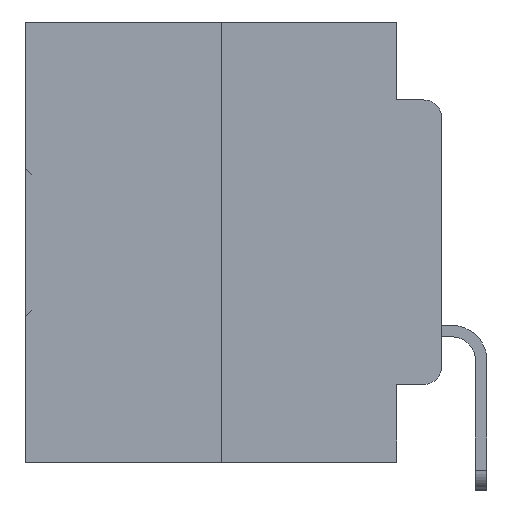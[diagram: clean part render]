
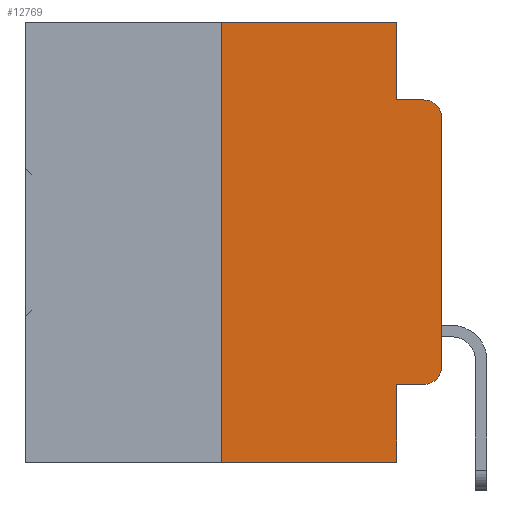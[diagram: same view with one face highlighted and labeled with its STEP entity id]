
A CAD part, left-side view. The second image highlights one B-rep face of the part: STEP entity #12769.
In plain terms, the highlighted planar face has unit normal (-1, 0, 0).
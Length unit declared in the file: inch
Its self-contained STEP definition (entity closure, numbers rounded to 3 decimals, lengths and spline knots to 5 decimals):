
#136 = CARTESIAN_POINT ( 'NONE',  ( 0., 0.02, -0.1085 ) ) ;
#420 = VECTOR ( 'NONE', #32712, 39.37008 ) ;
#559 = LINE ( 'NONE', #23580, #27703 ) ;
#702 = EDGE_CURVE ( 'NONE', #16581, #24952, #32642, .T. ) ;
#1032 = VERTEX_POINT ( 'NONE', #11957 ) ;
#1136 = CARTESIAN_POINT ( 'NONE',  ( 0., 0.02, -0.3915 ) ) ;
#1453 = ORIENTED_EDGE ( 'NONE', *, *, #24334, .T. ) ;
#2883 = DIRECTION ( 'NONE',  ( 0., 0., -1. ) ) ;
#3079 = ORIENTED_EDGE ( 'NONE', *, *, #13351, .F. ) ;
#3846 = DIRECTION ( 'NONE',  ( 0., 0., -1. ) ) ;
#4334 = EDGE_CURVE ( 'NONE', #1032, #16581, #8458, .T. ) ;
#4738 = EDGE_CURVE ( 'NONE', #27510, #22793, #20989, .T. ) ;
#4825 = EDGE_LOOP ( 'NONE', ( #1453, #26632, #18326, #22467, #15702, #8061, #13616, #3079, #13171, #13235 ) ) ;
#5275 = VECTOR ( 'NONE', #8597, 39.37008 ) ;
#6182 = VECTOR ( 'NONE', #15870, 39.37008 ) ;
#6198 = CARTESIAN_POINT ( 'NONE',  ( 0., 0.473, 0. ) ) ;
#6335 = AXIS2_PLACEMENT_3D ( 'NONE', #136, #18748, #2883 ) ;
#6555 = CARTESIAN_POINT ( 'NONE',  ( 0., 0.02, -0.0885 ) ) ;
#7232 = DIRECTION ( 'NONE',  ( 0., -1., 0. ) ) ;
#7271 = LINE ( 'NONE', #9336, #18768 ) ;
#7338 = LINE ( 'NONE', #14507, #20489 ) ;
#7946 = EDGE_CURVE ( 'NONE', #31544, #31928, #7271, .T. ) ;
#8061 = ORIENTED_EDGE ( 'NONE', *, *, #7946, .F. ) ;
#8458 = LINE ( 'NONE', #33052, #420 ) ;
#8597 = DIRECTION ( 'NONE',  ( 0., 0., -1. ) ) ;
#8681 = FACE_OUTER_BOUND ( 'NONE', #4825, .T. ) ;
#8871 = PLANE ( 'NONE',  #21609 ) ;
#9336 = CARTESIAN_POINT ( 'NONE',  ( 0., 0.25, 0. ) ) ;
#11580 = CARTESIAN_POINT ( 'NONE',  ( 0., 0.25, -0.5 ) ) ;
#11719 = CARTESIAN_POINT ( 'NONE',  ( 0., 0.02, -0.4115 ) ) ;
#11918 = AXIS2_PLACEMENT_3D ( 'NONE', #1136, #19691, #3846 ) ;
#11957 = CARTESIAN_POINT ( 'NONE',  ( 0., 0.051, 0. ) ) ;
#12186 = CARTESIAN_POINT ( 'NONE',  ( 0., 0., -0.1085 ) ) ;
#12450 = LINE ( 'NONE', #13882, #5275 ) ;
#12769 = ADVANCED_FACE ( 'NONE', ( #8681 ), #8871, .F. ) ;
#13171 = ORIENTED_EDGE ( 'NONE', *, *, #4738, .T. ) ;
#13235 = ORIENTED_EDGE ( 'NONE', *, *, #17181, .T. ) ;
#13351 = EDGE_CURVE ( 'NONE', #27510, #23651, #12450, .T. ) ;
#13353 = DIRECTION ( 'NONE',  ( 0., -1., 0. ) ) ;
#13616 = ORIENTED_EDGE ( 'NONE', *, *, #30329, .T. ) ;
#13882 = CARTESIAN_POINT ( 'NONE',  ( 0., 0.051, 0. ) ) ;
#14507 = CARTESIAN_POINT ( 'NONE',  ( 0., 0., 0. ) ) ;
#15702 = ORIENTED_EDGE ( 'NONE', *, *, #25125, .F. ) ;
#15870 = DIRECTION ( 'NONE',  ( 0., -1., 0. ) ) ;
#15890 = CARTESIAN_POINT ( 'NONE',  ( 0., 0.051, -0.4115 ) ) ;
#16581 = VERTEX_POINT ( 'NONE', #18728 ) ;
#16833 = DIRECTION ( 'NONE',  ( 0., 0., -1. ) ) ;
#17181 = EDGE_CURVE ( 'NONE', #22793, #25713, #19619, .T. ) ;
#17774 = VERTEX_POINT ( 'NONE', #12186 ) ;
#18326 = ORIENTED_EDGE ( 'NONE', *, *, #702, .F. ) ;
#18613 = CIRCLE ( 'NONE', #6335, 0.02 ) ;
#18728 = CARTESIAN_POINT ( 'NONE',  ( 0., 0.051, -0.0885 ) ) ;
#18748 = DIRECTION ( 'NONE',  ( -1., 0., 0. ) ) ;
#18768 = VECTOR ( 'NONE', #27503, 39.37008 ) ;
#19619 = CIRCLE ( 'NONE', #11918, 0.02 ) ;
#19691 = DIRECTION ( 'NONE',  ( -1., 0., 0. ) ) ;
#19696 = DIRECTION ( 'NONE',  ( 0., 0., 1. ) ) ;
#20489 = VECTOR ( 'NONE', #19696, 39.37008 ) ;
#20989 = LINE ( 'NONE', #15890, #6182 ) ;
#21609 = AXIS2_PLACEMENT_3D ( 'NONE', #6198, #32214, #16833 ) ;
#22467 = ORIENTED_EDGE ( 'NONE', *, *, #4334, .F. ) ;
#22793 = VERTEX_POINT ( 'NONE', #11719 ) ;
#23580 = CARTESIAN_POINT ( 'NONE',  ( 0., 0.473, -0.5 ) ) ;
#23651 = VERTEX_POINT ( 'NONE', #29346 ) ;
#24334 = EDGE_CURVE ( 'NONE', #25713, #17774, #7338, .T. ) ;
#24829 = DIRECTION ( 'NONE',  ( 0., -1., 0. ) ) ;
#24952 = VERTEX_POINT ( 'NONE', #6555 ) ;
#25125 = EDGE_CURVE ( 'NONE', #31928, #1032, #30451, .T. ) ;
#25713 = VERTEX_POINT ( 'NONE', #26547 ) ;
#25841 = VECTOR ( 'NONE', #24829, 39.37008 ) ;
#25899 = CARTESIAN_POINT ( 'NONE',  ( 0., 0.25, 0. ) ) ;
#26359 = CARTESIAN_POINT ( 'NONE',  ( 0., 0.051, -0.0885 ) ) ;
#26547 = CARTESIAN_POINT ( 'NONE',  ( 0., 0., -0.3915 ) ) ;
#26632 = ORIENTED_EDGE ( 'NONE', *, *, #27778, .T. ) ;
#27503 = DIRECTION ( 'NONE',  ( 0., 0., 1. ) ) ;
#27510 = VERTEX_POINT ( 'NONE', #27879 ) ;
#27703 = VECTOR ( 'NONE', #13353, 39.37008 ) ;
#27778 = EDGE_CURVE ( 'NONE', #17774, #24952, #18613, .T. ) ;
#27879 = CARTESIAN_POINT ( 'NONE',  ( 0., 0.051, -0.4115 ) ) ;
#28822 = VECTOR ( 'NONE', #7232, 39.37008 ) ;
#29346 = CARTESIAN_POINT ( 'NONE',  ( 0., 0.051, -0.5 ) ) ;
#30329 = EDGE_CURVE ( 'NONE', #31544, #23651, #559, .T. ) ;
#30451 = LINE ( 'NONE', #33185, #28822 ) ;
#31544 = VERTEX_POINT ( 'NONE', #11580 ) ;
#31928 = VERTEX_POINT ( 'NONE', #25899 ) ;
#32214 = DIRECTION ( 'NONE',  ( 1., 0., 0. ) ) ;
#32642 = LINE ( 'NONE', #26359, #25841 ) ;
#32712 = DIRECTION ( 'NONE',  ( 0., 0., -1. ) ) ;
#33052 = CARTESIAN_POINT ( 'NONE',  ( 0., 0.051, 0. ) ) ;
#33185 = CARTESIAN_POINT ( 'NONE',  ( 0., 0.473, 0. ) ) ;
